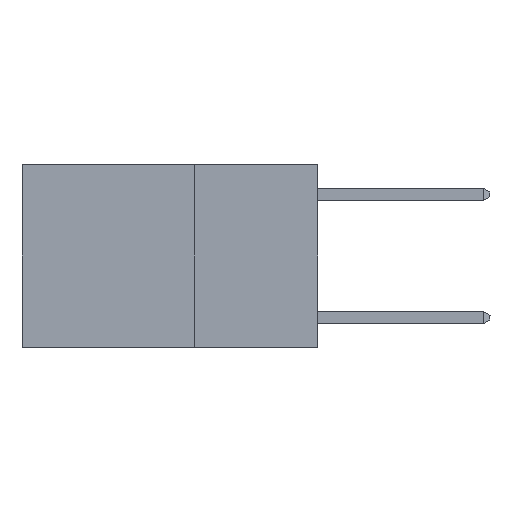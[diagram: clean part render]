
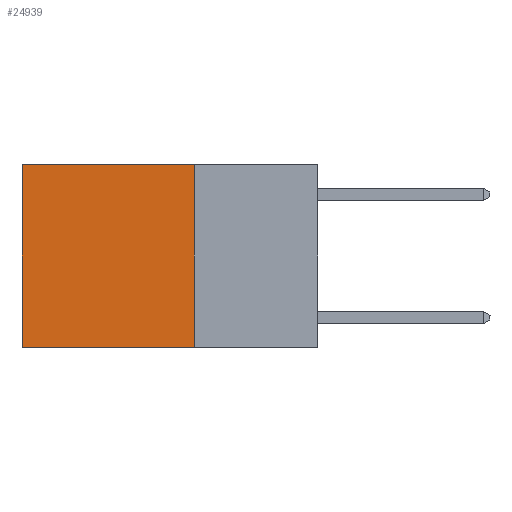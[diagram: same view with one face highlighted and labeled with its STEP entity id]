
A CAD part, left-side view. The second image highlights one B-rep face of the part: STEP entity #24939.
In plain terms, the highlighted planar face has unit normal (-1, 0, 0).
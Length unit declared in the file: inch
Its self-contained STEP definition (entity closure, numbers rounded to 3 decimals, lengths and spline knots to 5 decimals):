
#500 = EDGE_CURVE ( 'NONE', #19834, #17037, #6304, .T. ) ;
#1461 = VERTEX_POINT ( 'NONE', #24924 ) ;
#4564 = CARTESIAN_POINT ( 'NONE',  ( 0.2625, 0.25, -0.37 ) ) ;
#5384 = EDGE_CURVE ( 'NONE', #1461, #17037, #19373, .T. ) ;
#5555 = AXIS2_PLACEMENT_3D ( 'NONE', #21678, #9649, #23652 ) ;
#5608 = DIRECTION ( 'NONE',  ( 0., 0., -1. ) ) ;
#6304 = LINE ( 'NONE', #17844, #22408 ) ;
#9261 = VECTOR ( 'NONE', #24757, 39.37008 ) ;
#9649 = DIRECTION ( 'NONE',  ( 1., 0., 0. ) ) ;
#11294 = VERTEX_POINT ( 'NONE', #26018 ) ;
#13982 = LINE ( 'NONE', #20492, #23845 ) ;
#14337 = DIRECTION ( 'NONE',  ( 0., 0., -1. ) ) ;
#15912 = EDGE_LOOP ( 'NONE', ( #20018, #20386, #20533, #20737 ) ) ;
#16343 = CARTESIAN_POINT ( 'NONE',  ( 0.2625, 0.25, 0. ) ) ;
#17037 = VERTEX_POINT ( 'NONE', #24580 ) ;
#17844 = CARTESIAN_POINT ( 'NONE',  ( 0.2625, 0.6, 0. ) ) ;
#19373 = LINE ( 'NONE', #4564, #9261 ) ;
#19695 = PLANE ( 'NONE',  #5555 ) ;
#19834 = VERTEX_POINT ( 'NONE', #23924 ) ;
#20012 = EDGE_CURVE ( 'NONE', #11294, #19834, #13982, .T. ) ;
#20018 = ORIENTED_EDGE ( 'NONE', *, *, #500, .T. ) ;
#20386 = ORIENTED_EDGE ( 'NONE', *, *, #5384, .F. ) ;
#20492 = CARTESIAN_POINT ( 'NONE',  ( 0.2625, 0.25, 0. ) ) ;
#20533 = ORIENTED_EDGE ( 'NONE', *, *, #21767, .F. ) ;
#20726 = VECTOR ( 'NONE', #14337, 39.37008 ) ;
#20737 = ORIENTED_EDGE ( 'NONE', *, *, #20012, .T. ) ;
#21335 = LINE ( 'NONE', #16343, #20726 ) ;
#21678 = CARTESIAN_POINT ( 'NONE',  ( 0.2625, 0.25, 0. ) ) ;
#21767 = EDGE_CURVE ( 'NONE', #11294, #1461, #21335, .T. ) ;
#22408 = VECTOR ( 'NONE', #5608, 39.37008 ) ;
#22478 = DIRECTION ( 'NONE',  ( 0., 1., 0. ) ) ;
#23026 = FACE_OUTER_BOUND ( 'NONE', #15912, .T. ) ;
#23652 = DIRECTION ( 'NONE',  ( 0., 0., -1. ) ) ;
#23845 = VECTOR ( 'NONE', #22478, 39.37008 ) ;
#23924 = CARTESIAN_POINT ( 'NONE',  ( 0.2625, 0.6, 0. ) ) ;
#24580 = CARTESIAN_POINT ( 'NONE',  ( 0.2625, 0.6, -0.37 ) ) ;
#24757 = DIRECTION ( 'NONE',  ( 0., 1., 0. ) ) ;
#24924 = CARTESIAN_POINT ( 'NONE',  ( 0.2625, 0.25, -0.37 ) ) ;
#24939 = ADVANCED_FACE ( 'NONE', ( #23026 ), #19695, .F. ) ;
#26018 = CARTESIAN_POINT ( 'NONE',  ( 0.2625, 0.25, 0. ) ) ;
